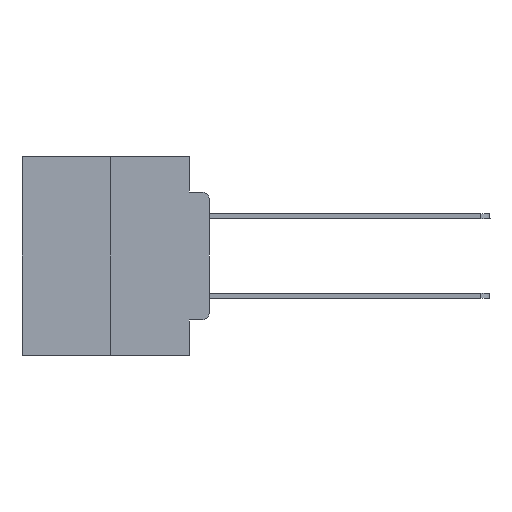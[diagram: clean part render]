
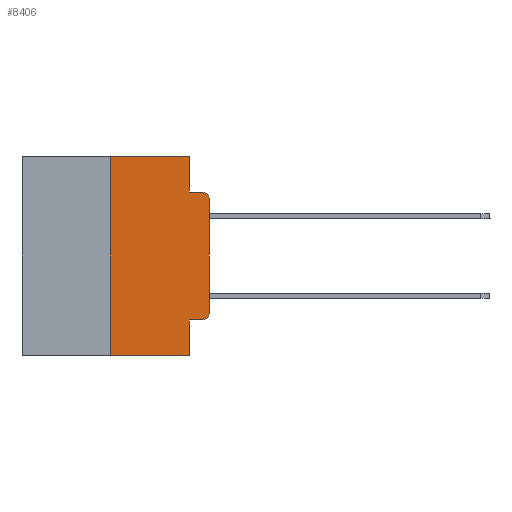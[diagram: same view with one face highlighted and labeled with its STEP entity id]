
A CAD part, left-side view. The second image highlights one B-rep face of the part: STEP entity #8406.
In plain terms, the highlighted planar face has unit normal (-1, 0, 0).
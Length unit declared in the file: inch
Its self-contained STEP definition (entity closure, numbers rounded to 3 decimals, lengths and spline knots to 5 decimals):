
#95 = AXIS2_PLACEMENT_3D ( 'NONE', #4559, #15114, #6413 ) ;
#363 = EDGE_CURVE ( 'NONE', #16704, #13397, #24667, .T. ) ;
#492 = VECTOR ( 'NONE', #6097, 39.37008 ) ;
#810 = CARTESIAN_POINT ( 'NONE',  ( 0., 0.02, -0.3915 ) ) ;
#873 = CARTESIAN_POINT ( 'NONE',  ( 0., 0.473, 0. ) ) ;
#1086 = VECTOR ( 'NONE', #4991, 39.37008 ) ;
#2050 = VECTOR ( 'NONE', #6426, 39.37008 ) ;
#2069 = CARTESIAN_POINT ( 'NONE',  ( 0., 0.02, -0.4115 ) ) ;
#2121 = VERTEX_POINT ( 'NONE', #12102 ) ;
#2291 = EDGE_CURVE ( 'NONE', #8004, #16704, #10544, .T. ) ;
#2354 = CARTESIAN_POINT ( 'NONE',  ( 0., 0., -0.1085 ) ) ;
#2586 = LINE ( 'NONE', #873, #1086 ) ;
#3222 = VERTEX_POINT ( 'NONE', #2354 ) ;
#3458 = CARTESIAN_POINT ( 'NONE',  ( 0., 0.02, -0.1085 ) ) ;
#3553 = CARTESIAN_POINT ( 'NONE',  ( 0., 0.051, 0. ) ) ;
#3810 = DIRECTION ( 'NONE',  ( 0., -1., 0. ) ) ;
#3870 = LINE ( 'NONE', #24045, #8761 ) ;
#4145 = FACE_OUTER_BOUND ( 'NONE', #21585, .T. ) ;
#4559 = CARTESIAN_POINT ( 'NONE',  ( 0., 0.473, 0. ) ) ;
#4991 = DIRECTION ( 'NONE',  ( 0., -1., 0. ) ) ;
#5302 = CARTESIAN_POINT ( 'NONE',  ( 0., 0., 0. ) ) ;
#5313 = ORIENTED_EDGE ( 'NONE', *, *, #23897, .T. ) ;
#5622 = ORIENTED_EDGE ( 'NONE', *, *, #363, .F. ) ;
#5734 = DIRECTION ( 'NONE',  ( 0., 0., -1. ) ) ;
#6097 = DIRECTION ( 'NONE',  ( 0., 0., -1. ) ) ;
#6278 = PLANE ( 'NONE',  #95 ) ;
#6373 = EDGE_CURVE ( 'NONE', #25724, #3222, #11874, .T. ) ;
#6413 = DIRECTION ( 'NONE',  ( 0., 0., -1. ) ) ;
#6426 = DIRECTION ( 'NONE',  ( 0., -1., 0. ) ) ;
#6718 = CARTESIAN_POINT ( 'NONE',  ( 0., 0.051, -0.5 ) ) ;
#7472 = AXIS2_PLACEMENT_3D ( 'NONE', #810, #12064, #22452 ) ;
#7571 = CIRCLE ( 'NONE', #24384, 0.02 ) ;
#8004 = VERTEX_POINT ( 'NONE', #27727 ) ;
#8406 = ADVANCED_FACE ( 'NONE', ( #4145 ), #6278, .F. ) ;
#8613 = VECTOR ( 'NONE', #22670, 39.37008 ) ;
#8761 = VECTOR ( 'NONE', #12560, 39.37008 ) ;
#8867 = CARTESIAN_POINT ( 'NONE',  ( 0., 0.02, -0.0885 ) ) ;
#9173 = ORIENTED_EDGE ( 'NONE', *, *, #12586, .T. ) ;
#10544 = LINE ( 'NONE', #3553, #492 ) ;
#11140 = LINE ( 'NONE', #17295, #2050 ) ;
#11874 = LINE ( 'NONE', #5302, #25384 ) ;
#11958 = CARTESIAN_POINT ( 'NONE',  ( 0., 0.25, 0. ) ) ;
#12064 = DIRECTION ( 'NONE',  ( -1., 0., 0. ) ) ;
#12102 = CARTESIAN_POINT ( 'NONE',  ( 0., 0.25, -0.5 ) ) ;
#12560 = DIRECTION ( 'NONE',  ( 0., 0., -1. ) ) ;
#12586 = EDGE_CURVE ( 'NONE', #12956, #25724, #20670, .T. ) ;
#12646 = LINE ( 'NONE', #14634, #17045 ) ;
#12956 = VERTEX_POINT ( 'NONE', #2069 ) ;
#13397 = VERTEX_POINT ( 'NONE', #8867 ) ;
#14213 = ORIENTED_EDGE ( 'NONE', *, *, #26322, .T. ) ;
#14334 = CARTESIAN_POINT ( 'NONE',  ( 0., 0., -0.3915 ) ) ;
#14634 = CARTESIAN_POINT ( 'NONE',  ( 0., 0.473, -0.5 ) ) ;
#14730 = VERTEX_POINT ( 'NONE', #19720 ) ;
#14761 = VERTEX_POINT ( 'NONE', #6718 ) ;
#15114 = DIRECTION ( 'NONE',  ( 1., 0., 0. ) ) ;
#16577 = ORIENTED_EDGE ( 'NONE', *, *, #6373, .T. ) ;
#16704 = VERTEX_POINT ( 'NONE', #17354 ) ;
#17023 = ORIENTED_EDGE ( 'NONE', *, *, #21974, .F. ) ;
#17045 = VECTOR ( 'NONE', #3810, 39.37008 ) ;
#17272 = ORIENTED_EDGE ( 'NONE', *, *, #2291, .F. ) ;
#17295 = CARTESIAN_POINT ( 'NONE',  ( 0., 0.051, -0.4115 ) ) ;
#17354 = CARTESIAN_POINT ( 'NONE',  ( 0., 0.051, -0.0885 ) ) ;
#17582 = VECTOR ( 'NONE', #22907, 39.37008 ) ;
#18297 = CARTESIAN_POINT ( 'NONE',  ( 0., 0.051, -0.0885 ) ) ;
#18823 = ORIENTED_EDGE ( 'NONE', *, *, #27035, .F. ) ;
#19082 = ORIENTED_EDGE ( 'NONE', *, *, #25074, .F. ) ;
#19720 = CARTESIAN_POINT ( 'NONE',  ( 0., 0.25, 0. ) ) ;
#20644 = LINE ( 'NONE', #11958, #17582 ) ;
#20670 = CIRCLE ( 'NONE', #7472, 0.02 ) ;
#20852 = DIRECTION ( 'NONE',  ( -1., 0., 0. ) ) ;
#21585 = EDGE_LOOP ( 'NONE', ( #16577, #23441, #5622, #17272, #19082, #18823, #5313, #17023, #14213, #9173 ) ) ;
#21974 = EDGE_CURVE ( 'NONE', #26283, #14761, #3870, .T. ) ;
#22452 = DIRECTION ( 'NONE',  ( 0., 0., -1. ) ) ;
#22670 = DIRECTION ( 'NONE',  ( 0., -1., 0. ) ) ;
#22907 = DIRECTION ( 'NONE',  ( 0., 0., 1. ) ) ;
#23441 = ORIENTED_EDGE ( 'NONE', *, *, #27505, .T. ) ;
#23897 = EDGE_CURVE ( 'NONE', #2121, #14761, #12646, .T. ) ;
#24045 = CARTESIAN_POINT ( 'NONE',  ( 0., 0.051, 0. ) ) ;
#24094 = CARTESIAN_POINT ( 'NONE',  ( 0., 0.051, -0.4115 ) ) ;
#24384 = AXIS2_PLACEMENT_3D ( 'NONE', #3458, #20852, #5734 ) ;
#24540 = DIRECTION ( 'NONE',  ( 0., 0., 1. ) ) ;
#24667 = LINE ( 'NONE', #18297, #8613 ) ;
#25074 = EDGE_CURVE ( 'NONE', #14730, #8004, #2586, .T. ) ;
#25384 = VECTOR ( 'NONE', #24540, 39.37008 ) ;
#25724 = VERTEX_POINT ( 'NONE', #14334 ) ;
#26283 = VERTEX_POINT ( 'NONE', #24094 ) ;
#26322 = EDGE_CURVE ( 'NONE', #26283, #12956, #11140, .T. ) ;
#27035 = EDGE_CURVE ( 'NONE', #2121, #14730, #20644, .T. ) ;
#27505 = EDGE_CURVE ( 'NONE', #3222, #13397, #7571, .T. ) ;
#27727 = CARTESIAN_POINT ( 'NONE',  ( 0., 0.051, 0. ) ) ;
